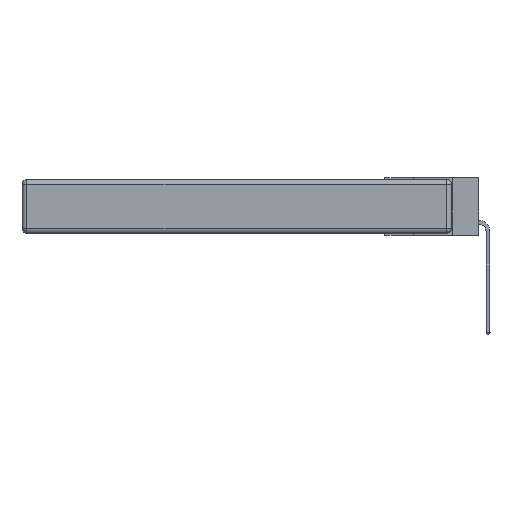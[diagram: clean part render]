
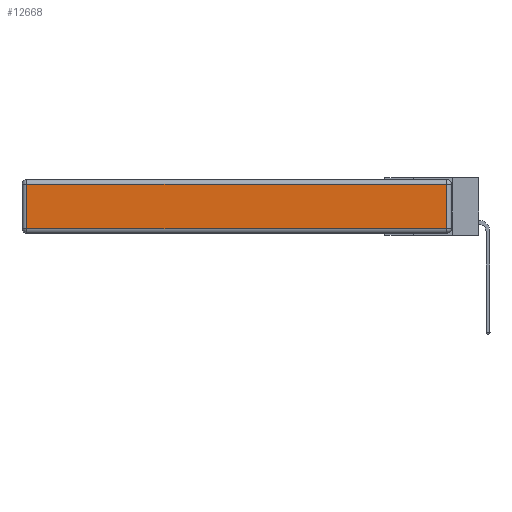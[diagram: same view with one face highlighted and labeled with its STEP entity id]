
A CAD part, left-side view. The second image highlights one B-rep face of the part: STEP entity #12668.
In plain terms, the highlighted planar face has unit normal (-1, 0, 0).
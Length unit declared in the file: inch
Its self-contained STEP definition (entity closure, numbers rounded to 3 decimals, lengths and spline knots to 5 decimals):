
#69 = CARTESIAN_POINT ( 'NONE',  ( 0., 0., -0.313 ) ) ;
#86 = LINE ( 'NONE', #69, #7484 ) ;
#199 = AXIS2_PLACEMENT_3D ( 'NONE', #5364, #426, #8292 ) ;
#221 = ORIENTED_EDGE ( 'NONE', *, *, #10011, .T. ) ;
#426 = DIRECTION ( 'NONE',  ( -1., 0., 0. ) ) ;
#623 = EDGE_CURVE ( 'NONE', #11195, #12378, #3847, .T. ) ;
#1349 = CARTESIAN_POINT ( 'NONE',  ( 0., 2.72, -0.343 ) ) ;
#1748 = FACE_OUTER_BOUND ( 'NONE', #4492, .T. ) ;
#2008 = LINE ( 'NONE', #10606, #5238 ) ;
#2366 = EDGE_CURVE ( 'NONE', #10535, #9463, #8706, .T. ) ;
#2489 = CARTESIAN_POINT ( 'NONE',  ( 0., 0.03, -0.313 ) ) ;
#2727 = VECTOR ( 'NONE', #3366, 39.37008 ) ;
#3366 = DIRECTION ( 'NONE',  ( 0., 0., -1. ) ) ;
#3847 = LINE ( 'NONE', #5591, #4008 ) ;
#4008 = VECTOR ( 'NONE', #12581, 39.37008 ) ;
#4492 = EDGE_LOOP ( 'NONE', ( #221, #9931, #7296, #8885 ) ) ;
#5238 = VECTOR ( 'NONE', #8574, 39.37008 ) ;
#5364 = CARTESIAN_POINT ( 'NONE',  ( 0., 0., -0.343 ) ) ;
#5591 = CARTESIAN_POINT ( 'NONE',  ( 0., 0.03, -0.343 ) ) ;
#6914 = EDGE_CURVE ( 'NONE', #12378, #10535, #2008, .T. ) ;
#7296 = ORIENTED_EDGE ( 'NONE', *, *, #6914, .T. ) ;
#7484 = VECTOR ( 'NONE', #12669, 39.37008 ) ;
#8253 = PLANE ( 'NONE',  #199 ) ;
#8292 = DIRECTION ( 'NONE',  ( 0., 0., 1. ) ) ;
#8401 = CARTESIAN_POINT ( 'NONE',  ( 0., 0.03, -0.03 ) ) ;
#8574 = DIRECTION ( 'NONE',  ( 0., 1., 0. ) ) ;
#8706 = LINE ( 'NONE', #1349, #2727 ) ;
#8885 = ORIENTED_EDGE ( 'NONE', *, *, #2366, .T. ) ;
#9463 = VERTEX_POINT ( 'NONE', #10881 ) ;
#9521 = CARTESIAN_POINT ( 'NONE',  ( 0., 2.72, -0.03 ) ) ;
#9931 = ORIENTED_EDGE ( 'NONE', *, *, #623, .T. ) ;
#10011 = EDGE_CURVE ( 'NONE', #9463, #11195, #86, .T. ) ;
#10535 = VERTEX_POINT ( 'NONE', #9521 ) ;
#10606 = CARTESIAN_POINT ( 'NONE',  ( 0., 2.75, -0.03 ) ) ;
#10881 = CARTESIAN_POINT ( 'NONE',  ( 0., 2.72, -0.313 ) ) ;
#11195 = VERTEX_POINT ( 'NONE', #2489 ) ;
#12378 = VERTEX_POINT ( 'NONE', #8401 ) ;
#12581 = DIRECTION ( 'NONE',  ( 0., 0., 1. ) ) ;
#12668 = ADVANCED_FACE ( 'NONE', ( #1748 ), #8253, .T. ) ;
#12669 = DIRECTION ( 'NONE',  ( 0., -1., 0. ) ) ;
